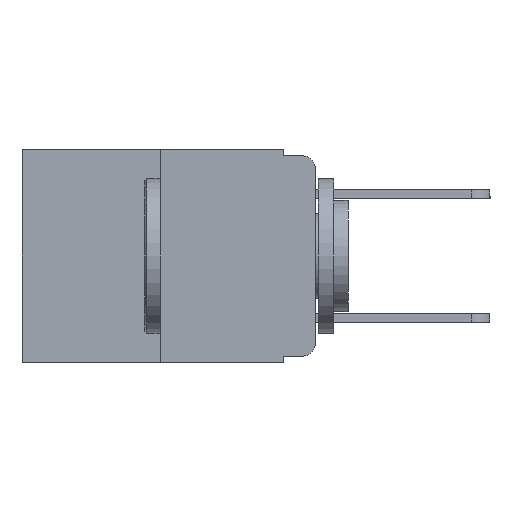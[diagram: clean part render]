
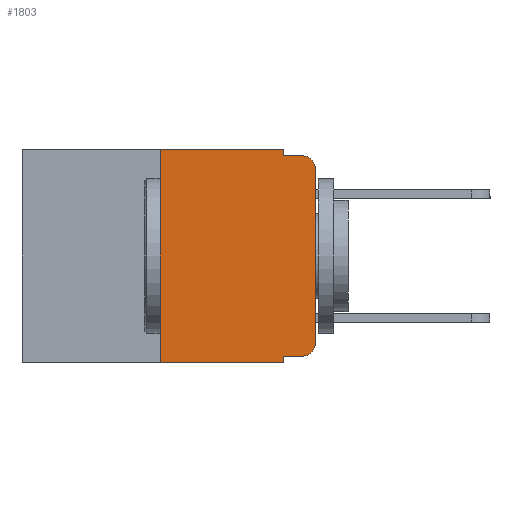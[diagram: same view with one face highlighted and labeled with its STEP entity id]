
A CAD part, left-side view. The second image highlights one B-rep face of the part: STEP entity #1803.
In plain terms, the highlighted planar face has unit normal (-1, 0, 0).
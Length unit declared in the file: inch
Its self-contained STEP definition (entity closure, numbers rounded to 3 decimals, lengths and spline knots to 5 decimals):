
#76 = DIRECTION ( 'NONE',  ( 0., -1., 0. ) ) ;
#380 = VERTEX_POINT ( 'NONE', #15976 ) ;
#540 = VECTOR ( 'NONE', #4523, 39.37008 ) ;
#787 = DIRECTION ( 'NONE',  ( 0., 0., -1. ) ) ;
#1045 = CARTESIAN_POINT ( 'NONE',  ( 0., 0., 0. ) ) ;
#1332 = EDGE_CURVE ( 'NONE', #3924, #7978, #7632, .T. ) ;
#1376 = ORIENTED_EDGE ( 'NONE', *, *, #12162, .T. ) ;
#1803 = ADVANCED_FACE ( 'NONE', ( #14146 ), #9396, .F. ) ;
#1811 = DIRECTION ( 'NONE',  ( 0., 0., -1. ) ) ;
#2199 = VERTEX_POINT ( 'NONE', #7282 ) ;
#2464 = VERTEX_POINT ( 'NONE', #13437 ) ;
#2759 = LINE ( 'NONE', #4446, #12303 ) ;
#2785 = ORIENTED_EDGE ( 'NONE', *, *, #8256, .T. ) ;
#3468 = EDGE_CURVE ( 'NONE', #7978, #15438, #16475, .T. ) ;
#3767 = CARTESIAN_POINT ( 'NONE',  ( 0., 0.02, -0.01 ) ) ;
#3847 = ORIENTED_EDGE ( 'NONE', *, *, #10462, .T. ) ;
#3924 = VERTEX_POINT ( 'NONE', #14818 ) ;
#4167 = DIRECTION ( 'NONE',  ( 0., 0., -1. ) ) ;
#4198 = DIRECTION ( 'NONE',  ( 1., 0., 0. ) ) ;
#4386 = LINE ( 'NONE', #12237, #16438 ) ;
#4446 = CARTESIAN_POINT ( 'NONE',  ( 0., 0.473, 0. ) ) ;
#4523 = DIRECTION ( 'NONE',  ( 0., -1., 0. ) ) ;
#4839 = VERTEX_POINT ( 'NONE', #11957 ) ;
#4872 = ORIENTED_EDGE ( 'NONE', *, *, #5314, .T. ) ;
#4893 = VERTEX_POINT ( 'NONE', #12051 ) ;
#5019 = LINE ( 'NONE', #16535, #540 ) ;
#5128 = CIRCLE ( 'NONE', #15808, 0.02 ) ;
#5267 = ORIENTED_EDGE ( 'NONE', *, *, #3468, .F. ) ;
#5314 = EDGE_CURVE ( 'NONE', #380, #15438, #12293, .T. ) ;
#5470 = LINE ( 'NONE', #1045, #8913 ) ;
#5503 = VERTEX_POINT ( 'NONE', #15157 ) ;
#5650 = VERTEX_POINT ( 'NONE', #8461 ) ;
#6029 = ORIENTED_EDGE ( 'NONE', *, *, #1332, .F. ) ;
#6248 = AXIS2_PLACEMENT_3D ( 'NONE', #7605, #4198, #4167 ) ;
#6828 = DIRECTION ( 'NONE',  ( 0., 0., 1. ) ) ;
#6878 = DIRECTION ( 'NONE',  ( -1., 0., 0. ) ) ;
#7282 = CARTESIAN_POINT ( 'NONE',  ( 0., 0.25, 0. ) ) ;
#7370 = ORIENTED_EDGE ( 'NONE', *, *, #15322, .F. ) ;
#7451 = EDGE_LOOP ( 'NONE', ( #3847, #4872, #5267, #6029, #8511, #7370, #1376, #14330, #13217, #2785 ) ) ;
#7457 = VECTOR ( 'NONE', #11290, 39.37008 ) ;
#7605 = CARTESIAN_POINT ( 'NONE',  ( 0., 0.473, 0. ) ) ;
#7632 = LINE ( 'NONE', #12860, #10930 ) ;
#7978 = VERTEX_POINT ( 'NONE', #12582 ) ;
#8256 = EDGE_CURVE ( 'NONE', #4893, #5650, #5128, .T. ) ;
#8345 = VECTOR ( 'NONE', #15408, 39.37008 ) ;
#8461 = CARTESIAN_POINT ( 'NONE',  ( 0., 0., -0.313 ) ) ;
#8511 = ORIENTED_EDGE ( 'NONE', *, *, #10635, .F. ) ;
#8567 = CARTESIAN_POINT ( 'NONE',  ( 0., 0.051, -0.01 ) ) ;
#8913 = VECTOR ( 'NONE', #6828, 39.37008 ) ;
#9132 = DIRECTION ( 'NONE',  ( -1., 0., 0. ) ) ;
#9396 = PLANE ( 'NONE',  #6248 ) ;
#9472 = LINE ( 'NONE', #11229, #15259 ) ;
#10102 = CARTESIAN_POINT ( 'NONE',  ( 0., 0.25, 0. ) ) ;
#10462 = EDGE_CURVE ( 'NONE', #5650, #380, #5470, .T. ) ;
#10635 = EDGE_CURVE ( 'NONE', #2199, #3924, #2759, .T. ) ;
#10757 = EDGE_CURVE ( 'NONE', #2464, #4893, #4386, .T. ) ;
#10930 = VECTOR ( 'NONE', #1811, 39.37008 ) ;
#11229 = CARTESIAN_POINT ( 'NONE',  ( 0., 0.051, 0. ) ) ;
#11290 = DIRECTION ( 'NONE',  ( 0., 0., 1. ) ) ;
#11957 = CARTESIAN_POINT ( 'NONE',  ( 0., 0.25, -0.343 ) ) ;
#12051 = CARTESIAN_POINT ( 'NONE',  ( 0., 0.02, -0.333 ) ) ;
#12162 = EDGE_CURVE ( 'NONE', #4839, #5503, #5019, .T. ) ;
#12237 = CARTESIAN_POINT ( 'NONE',  ( 0., 0.051, -0.333 ) ) ;
#12293 = CIRCLE ( 'NONE', #15972, 0.02 ) ;
#12303 = VECTOR ( 'NONE', #14294, 39.37008 ) ;
#12407 = DIRECTION ( 'NONE',  ( 0., 0., -1. ) ) ;
#12582 = CARTESIAN_POINT ( 'NONE',  ( 0., 0.051, -0.01 ) ) ;
#12860 = CARTESIAN_POINT ( 'NONE',  ( 0., 0.051, 0. ) ) ;
#13217 = ORIENTED_EDGE ( 'NONE', *, *, #10757, .T. ) ;
#13437 = CARTESIAN_POINT ( 'NONE',  ( 0., 0.051, -0.333 ) ) ;
#13848 = EDGE_CURVE ( 'NONE', #2464, #5503, #9472, .T. ) ;
#14094 = CARTESIAN_POINT ( 'NONE',  ( 0., 0.02, -0.313 ) ) ;
#14146 = FACE_OUTER_BOUND ( 'NONE', #7451, .T. ) ;
#14188 = LINE ( 'NONE', #10102, #7457 ) ;
#14294 = DIRECTION ( 'NONE',  ( 0., -1., 0. ) ) ;
#14330 = ORIENTED_EDGE ( 'NONE', *, *, #13848, .F. ) ;
#14818 = CARTESIAN_POINT ( 'NONE',  ( 0., 0.051, 0. ) ) ;
#15157 = CARTESIAN_POINT ( 'NONE',  ( 0., 0.051, -0.343 ) ) ;
#15196 = DIRECTION ( 'NONE',  ( 0., 0., -1. ) ) ;
#15259 = VECTOR ( 'NONE', #12407, 39.37008 ) ;
#15322 = EDGE_CURVE ( 'NONE', #4839, #2199, #14188, .T. ) ;
#15408 = DIRECTION ( 'NONE',  ( 0., -1., 0. ) ) ;
#15438 = VERTEX_POINT ( 'NONE', #3767 ) ;
#15808 = AXIS2_PLACEMENT_3D ( 'NONE', #14094, #6878, #15196 ) ;
#15972 = AXIS2_PLACEMENT_3D ( 'NONE', #16035, #9132, #787 ) ;
#15976 = CARTESIAN_POINT ( 'NONE',  ( 0., 0., -0.03 ) ) ;
#16035 = CARTESIAN_POINT ( 'NONE',  ( 0., 0.02, -0.03 ) ) ;
#16438 = VECTOR ( 'NONE', #76, 39.37008 ) ;
#16475 = LINE ( 'NONE', #8567, #8345 ) ;
#16535 = CARTESIAN_POINT ( 'NONE',  ( 0., 0.473, -0.343 ) ) ;
